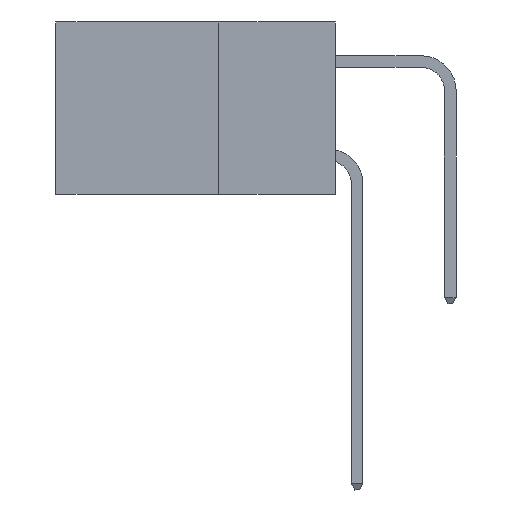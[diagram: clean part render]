
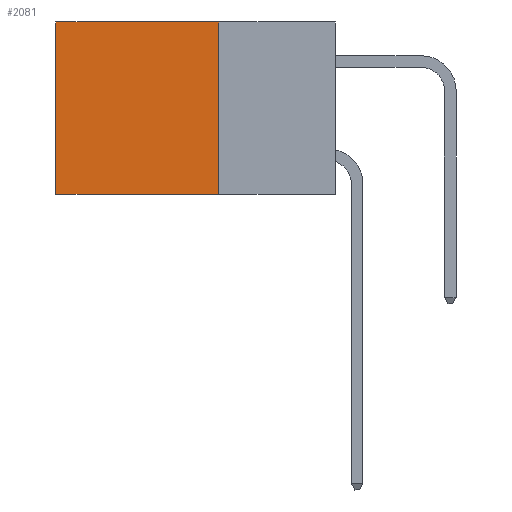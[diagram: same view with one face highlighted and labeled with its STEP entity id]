
A CAD part, left-side view. The second image highlights one B-rep face of the part: STEP entity #2081.
In plain terms, the highlighted planar face has unit normal (-1, 0, 0).
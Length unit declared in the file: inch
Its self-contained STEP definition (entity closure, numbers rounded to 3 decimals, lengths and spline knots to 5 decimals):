
#222 = CARTESIAN_POINT ( 'NONE',  ( 0.2875, 0.6, -0.37 ) ) ;
#617 = DIRECTION ( 'NONE',  ( 0., 1., 0. ) ) ;
#2081 = ADVANCED_FACE ( 'NONE', ( #20810 ), #29361, .F. ) ;
#2239 = EDGE_LOOP ( 'NONE', ( #3401, #24133, #14799, #20977 ) ) ;
#3310 = CARTESIAN_POINT ( 'NONE',  ( 0.2875, 0.25, -0.37 ) ) ;
#3401 = ORIENTED_EDGE ( 'NONE', *, *, #19861, .T. ) ;
#8583 = DIRECTION ( 'NONE',  ( 0., 0., -1. ) ) ;
#9352 = CARTESIAN_POINT ( 'NONE',  ( 0.2875, 0.6, 0. ) ) ;
#11297 = LINE ( 'NONE', #23956, #31367 ) ;
#12791 = VECTOR ( 'NONE', #20080, 39.37008 ) ;
#12968 = CARTESIAN_POINT ( 'NONE',  ( 0.2875, 0.25, 0. ) ) ;
#13721 = CARTESIAN_POINT ( 'NONE',  ( 0.2875, 0.25, 0. ) ) ;
#14422 = AXIS2_PLACEMENT_3D ( 'NONE', #13721, #21521, #8583 ) ;
#14429 = VERTEX_POINT ( 'NONE', #3310 ) ;
#14791 = CARTESIAN_POINT ( 'NONE',  ( 0.2875, 0.25, 0. ) ) ;
#14799 = ORIENTED_EDGE ( 'NONE', *, *, #23380, .F. ) ;
#15227 = CARTESIAN_POINT ( 'NONE',  ( 0.2875, 0.25, -0.37 ) ) ;
#17442 = EDGE_CURVE ( 'NONE', #14429, #24954, #29380, .T. ) ;
#18211 = VERTEX_POINT ( 'NONE', #9352 ) ;
#19738 = LINE ( 'NONE', #12968, #12791 ) ;
#19861 = EDGE_CURVE ( 'NONE', #18211, #24954, #20391, .T. ) ;
#20080 = DIRECTION ( 'NONE',  ( 0., 0., -1. ) ) ;
#20391 = LINE ( 'NONE', #24491, #33413 ) ;
#20810 = FACE_OUTER_BOUND ( 'NONE', #2239, .T. ) ;
#20977 = ORIENTED_EDGE ( 'NONE', *, *, #24956, .T. ) ;
#21521 = DIRECTION ( 'NONE',  ( 1., 0., 0. ) ) ;
#22488 = VECTOR ( 'NONE', #28423, 39.37008 ) ;
#23380 = EDGE_CURVE ( 'NONE', #25259, #14429, #19738, .T. ) ;
#23956 = CARTESIAN_POINT ( 'NONE',  ( 0.2875, 0.25, 0. ) ) ;
#24133 = ORIENTED_EDGE ( 'NONE', *, *, #17442, .F. ) ;
#24491 = CARTESIAN_POINT ( 'NONE',  ( 0.2875, 0.6, 0. ) ) ;
#24954 = VERTEX_POINT ( 'NONE', #222 ) ;
#24956 = EDGE_CURVE ( 'NONE', #25259, #18211, #11297, .T. ) ;
#25259 = VERTEX_POINT ( 'NONE', #14791 ) ;
#28423 = DIRECTION ( 'NONE',  ( 0., 1., 0. ) ) ;
#29361 = PLANE ( 'NONE',  #14422 ) ;
#29380 = LINE ( 'NONE', #15227, #22488 ) ;
#29707 = DIRECTION ( 'NONE',  ( 0., 0., -1. ) ) ;
#31367 = VECTOR ( 'NONE', #617, 39.37008 ) ;
#33413 = VECTOR ( 'NONE', #29707, 39.37008 ) ;
